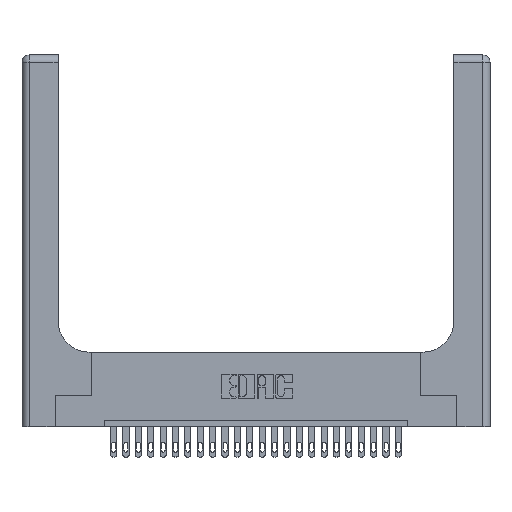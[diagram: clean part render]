
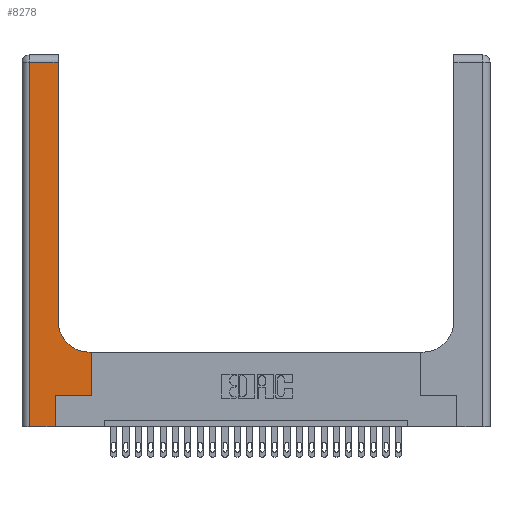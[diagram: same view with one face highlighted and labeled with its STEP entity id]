
A CAD part, top view. The second image highlights one B-rep face of the part: STEP entity #8278.
In plain terms, the highlighted planar face has unit normal (0, 0, 1).
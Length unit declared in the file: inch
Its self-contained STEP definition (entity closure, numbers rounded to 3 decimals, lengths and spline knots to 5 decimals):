
#977 = CARTESIAN_POINT ( 'NONE',  ( 0.269, 0.25, 0.37 ) ) ;
#1076 = VERTEX_POINT ( 'NONE', #12197 ) ;
#1313 = VECTOR ( 'NONE', #17451, 39.37008 ) ;
#1770 = VERTEX_POINT ( 'NONE', #21566 ) ;
#1938 = VERTEX_POINT ( 'NONE', #23816 ) ;
#2207 = LINE ( 'NONE', #7306, #1313 ) ;
#2472 = LINE ( 'NONE', #25094, #24442 ) ;
#2808 = EDGE_CURVE ( 'NONE', #19698, #25563, #17786, .T. ) ;
#3183 = VECTOR ( 'NONE', #19055, 39.37008 ) ;
#3309 = ORIENTED_EDGE ( 'NONE', *, *, #25508, .T. ) ;
#3446 = ORIENTED_EDGE ( 'NONE', *, *, #8933, .T. ) ;
#4393 = EDGE_LOOP ( 'NONE', ( #6323, #16524, #6439, #12173, #15391, #12065, #22101, #3446, #3309 ) ) ;
#4428 = VECTOR ( 'NONE', #6560, 39.37008 ) ;
#5098 = FACE_OUTER_BOUND ( 'NONE', #4393, .T. ) ;
#5167 = CARTESIAN_POINT ( 'NONE',  ( 0.06, 0., 0.37 ) ) ;
#5777 = AXIS2_PLACEMENT_3D ( 'NONE', #24360, #16760, #6524 ) ;
#6323 = ORIENTED_EDGE ( 'NONE', *, *, #12816, .T. ) ;
#6439 = ORIENTED_EDGE ( 'NONE', *, *, #21012, .T. ) ;
#6524 = DIRECTION ( 'NONE',  ( -1., 0., 0. ) ) ;
#6560 = DIRECTION ( 'NONE',  ( 1., 0., 0. ) ) ;
#6617 = CARTESIAN_POINT ( 'NONE',  ( 0.2915, 0.6, 0.37 ) ) ;
#7271 = VECTOR ( 'NONE', #7983, 39.37008 ) ;
#7306 = CARTESIAN_POINT ( 'NONE',  ( 0., 2.94, 0.37 ) ) ;
#7941 = CIRCLE ( 'NONE', #21922, 0.25 ) ;
#7983 = DIRECTION ( 'NONE',  ( -1., 0., 0. ) ) ;
#8278 = ADVANCED_FACE ( 'NONE', ( #5098 ), #16421, .F. ) ;
#8373 = EDGE_CURVE ( 'NONE', #14208, #19698, #12265, .T. ) ;
#8470 = DIRECTION ( 'NONE',  ( 0., 1., 0. ) ) ;
#8933 = EDGE_CURVE ( 'NONE', #1770, #1076, #9462, .T. ) ;
#8972 = LINE ( 'NONE', #25346, #24764 ) ;
#9025 = VECTOR ( 'NONE', #17414, 39.37008 ) ;
#9462 = LINE ( 'NONE', #6617, #7271 ) ;
#10839 = CARTESIAN_POINT ( 'NONE',  ( 0.2915, 2.94, 0.37 ) ) ;
#11558 = VERTEX_POINT ( 'NONE', #16045 ) ;
#11825 = VERTEX_POINT ( 'NONE', #5167 ) ;
#12065 = ORIENTED_EDGE ( 'NONE', *, *, #2808, .T. ) ;
#12173 = ORIENTED_EDGE ( 'NONE', *, *, #14958, .T. ) ;
#12197 = CARTESIAN_POINT ( 'NONE',  ( 0.5415, 0.6, 0.37 ) ) ;
#12265 = LINE ( 'NONE', #20277, #20300 ) ;
#12816 = EDGE_CURVE ( 'NONE', #11558, #22173, #2472, .T. ) ;
#13469 = EDGE_CURVE ( 'NONE', #22173, #1938, #2207, .T. ) ;
#14011 = CARTESIAN_POINT ( 'NONE',  ( 0.5585, 0.25, 0.37 ) ) ;
#14208 = VERTEX_POINT ( 'NONE', #16043 ) ;
#14805 = CARTESIAN_POINT ( 'NONE',  ( 0.269, 0.25, 0.37 ) ) ;
#14958 = EDGE_CURVE ( 'NONE', #11825, #14208, #8972, .T. ) ;
#15391 = ORIENTED_EDGE ( 'NONE', *, *, #8373, .T. ) ;
#16043 = CARTESIAN_POINT ( 'NONE',  ( 0.269, 0., 0.37 ) ) ;
#16045 = CARTESIAN_POINT ( 'NONE',  ( 0.2915, 0.85, 0.37 ) ) ;
#16421 = PLANE ( 'NONE',  #5777 ) ;
#16524 = ORIENTED_EDGE ( 'NONE', *, *, #13469, .T. ) ;
#16690 = CARTESIAN_POINT ( 'NONE',  ( 0.06, 3., 0.37 ) ) ;
#16760 = DIRECTION ( 'NONE',  ( 0., 0., -1. ) ) ;
#17414 = DIRECTION ( 'NONE',  ( 0., 1., 0. ) ) ;
#17451 = DIRECTION ( 'NONE',  ( -1., 0., 0. ) ) ;
#17786 = LINE ( 'NONE', #14805, #4428 ) ;
#18347 = DIRECTION ( 'NONE',  ( 1., 0., 0. ) ) ;
#19055 = DIRECTION ( 'NONE',  ( 0., -1., 0. ) ) ;
#19698 = VERTEX_POINT ( 'NONE', #977 ) ;
#20277 = CARTESIAN_POINT ( 'NONE',  ( 0.269, 0., 0.37 ) ) ;
#20300 = VECTOR ( 'NONE', #8470, 39.37008 ) ;
#20483 = CARTESIAN_POINT ( 'NONE',  ( 0.5415, 0.85, 0.37 ) ) ;
#20566 = LINE ( 'NONE', #16690, #3183 ) ;
#21012 = EDGE_CURVE ( 'NONE', #1938, #11825, #20566, .T. ) ;
#21138 = LINE ( 'NONE', #25171, #9025 ) ;
#21415 = DIRECTION ( 'NONE',  ( 0., 1., 0. ) ) ;
#21566 = CARTESIAN_POINT ( 'NONE',  ( 0.5585, 0.6, 0.37 ) ) ;
#21922 = AXIS2_PLACEMENT_3D ( 'NONE', #20483, #22127, #22211 ) ;
#22101 = ORIENTED_EDGE ( 'NONE', *, *, #22983, .T. ) ;
#22127 = DIRECTION ( 'NONE',  ( 0., 0., -1. ) ) ;
#22173 = VERTEX_POINT ( 'NONE', #10839 ) ;
#22211 = DIRECTION ( 'NONE',  ( 1., 0., 0. ) ) ;
#22983 = EDGE_CURVE ( 'NONE', #25563, #1770, #21138, .T. ) ;
#23816 = CARTESIAN_POINT ( 'NONE',  ( 0.06, 2.94, 0.37 ) ) ;
#24360 = CARTESIAN_POINT ( 'NONE',  ( 0., 3., 0.37 ) ) ;
#24442 = VECTOR ( 'NONE', #21415, 39.37008 ) ;
#24764 = VECTOR ( 'NONE', #18347, 39.37008 ) ;
#25094 = CARTESIAN_POINT ( 'NONE',  ( 0.2915, 3., 0.37 ) ) ;
#25171 = CARTESIAN_POINT ( 'NONE',  ( 0.5585, 0.25, 0.37 ) ) ;
#25346 = CARTESIAN_POINT ( 'NONE',  ( 0., 0., 0.37 ) ) ;
#25508 = EDGE_CURVE ( 'NONE', #1076, #11558, #7941, .T. ) ;
#25563 = VERTEX_POINT ( 'NONE', #14011 ) ;
